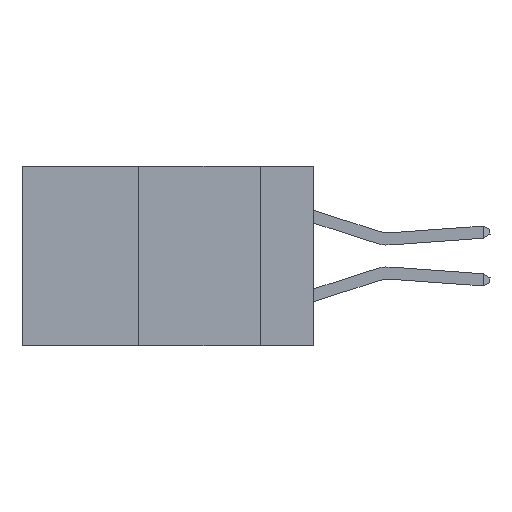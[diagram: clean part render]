
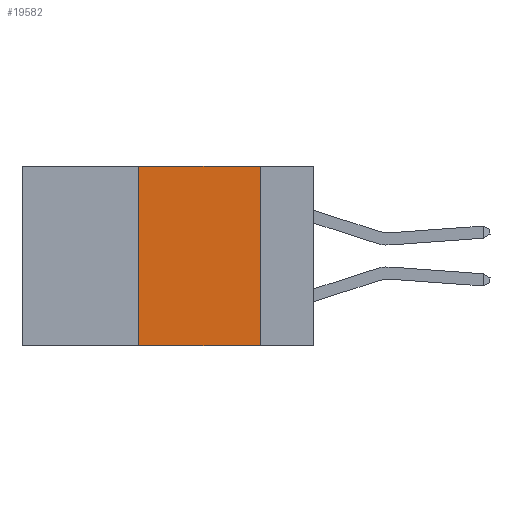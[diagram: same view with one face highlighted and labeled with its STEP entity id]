
A CAD part, left-side view. The second image highlights one B-rep face of the part: STEP entity #19582.
In plain terms, the highlighted planar face has unit normal (-1, 0, 0).
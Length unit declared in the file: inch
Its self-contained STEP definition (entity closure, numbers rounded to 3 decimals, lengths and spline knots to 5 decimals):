
#198 = CARTESIAN_POINT ( 'NONE',  ( 0., 0.11, 0. ) ) ;
#576 = ORIENTED_EDGE ( 'NONE', *, *, #22129, .T. ) ;
#894 = CARTESIAN_POINT ( 'NONE',  ( 0., 0.11, -0.37 ) ) ;
#2318 = VECTOR ( 'NONE', #11252, 39.37008 ) ;
#5306 = CARTESIAN_POINT ( 'NONE',  ( 0., 0.6, 0. ) ) ;
#5380 = CARTESIAN_POINT ( 'NONE',  ( 0., 0.6, -0.37 ) ) ;
#5827 = CARTESIAN_POINT ( 'NONE',  ( 0., 0.36, -0.37 ) ) ;
#5830 = VERTEX_POINT ( 'NONE', #14353 ) ;
#8118 = VERTEX_POINT ( 'NONE', #5827 ) ;
#8799 = EDGE_CURVE ( 'NONE', #5830, #24329, #14051, .T. ) ;
#10101 = LINE ( 'NONE', #5380, #17169 ) ;
#10646 = DIRECTION ( 'NONE',  ( 1., 0., 0. ) ) ;
#10685 = VECTOR ( 'NONE', #32309, 39.37008 ) ;
#10694 = ORIENTED_EDGE ( 'NONE', *, *, #18420, .F. ) ;
#11117 = DIRECTION ( 'NONE',  ( 0., -1., 0. ) ) ;
#11252 = DIRECTION ( 'NONE',  ( 0., 0., -1. ) ) ;
#11916 = VERTEX_POINT ( 'NONE', #894 ) ;
#14051 = LINE ( 'NONE', #26908, #34249 ) ;
#14353 = CARTESIAN_POINT ( 'NONE',  ( 0., 0.36, 0. ) ) ;
#15706 = LINE ( 'NONE', #27048, #2318 ) ;
#17169 = VECTOR ( 'NONE', #21214, 39.37008 ) ;
#18420 = EDGE_CURVE ( 'NONE', #24329, #11916, #15706, .T. ) ;
#18552 = ORIENTED_EDGE ( 'NONE', *, *, #8799, .F. ) ;
#19582 = ADVANCED_FACE ( 'NONE', ( #28866 ), #26429, .F. ) ;
#19715 = EDGE_CURVE ( 'NONE', #8118, #5830, #32553, .T. ) ;
#21214 = DIRECTION ( 'NONE',  ( 0., -1., 0. ) ) ;
#22129 = EDGE_CURVE ( 'NONE', #8118, #11916, #10101, .T. ) ;
#24329 = VERTEX_POINT ( 'NONE', #198 ) ;
#26381 = ORIENTED_EDGE ( 'NONE', *, *, #19715, .F. ) ;
#26429 = PLANE ( 'NONE',  #27598 ) ;
#26908 = CARTESIAN_POINT ( 'NONE',  ( 0., 0.6, 0. ) ) ;
#27048 = CARTESIAN_POINT ( 'NONE',  ( 0., 0.11, 0. ) ) ;
#27598 = AXIS2_PLACEMENT_3D ( 'NONE', #5306, #10646, #29098 ) ;
#28866 = FACE_OUTER_BOUND ( 'NONE', #31234, .T. ) ;
#29098 = DIRECTION ( 'NONE',  ( 0., 0., -1. ) ) ;
#29654 = CARTESIAN_POINT ( 'NONE',  ( 0., 0.36, 0. ) ) ;
#31234 = EDGE_LOOP ( 'NONE', ( #10694, #18552, #26381, #576 ) ) ;
#32309 = DIRECTION ( 'NONE',  ( 0., 0., 1. ) ) ;
#32553 = LINE ( 'NONE', #29654, #10685 ) ;
#34249 = VECTOR ( 'NONE', #11117, 39.37008 ) ;
